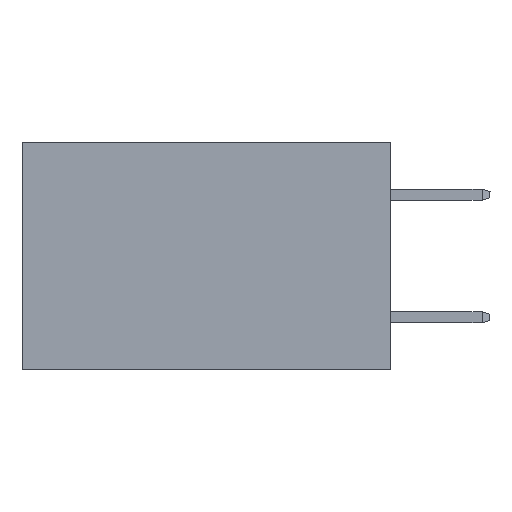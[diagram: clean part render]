
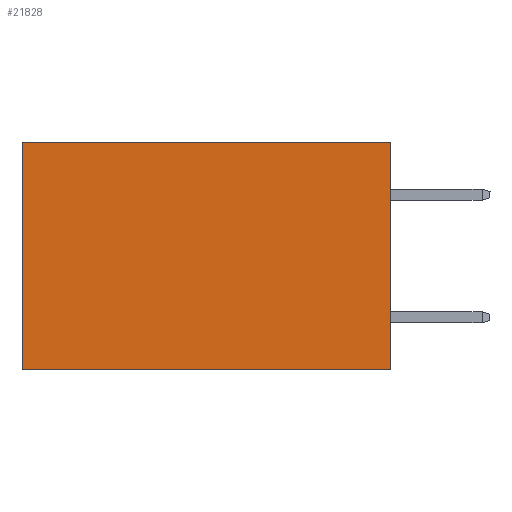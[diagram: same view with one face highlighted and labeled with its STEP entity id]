
A CAD part, left-side view. The second image highlights one B-rep face of the part: STEP entity #21828.
In plain terms, the highlighted planar face has unit normal (-1, 0, 0).
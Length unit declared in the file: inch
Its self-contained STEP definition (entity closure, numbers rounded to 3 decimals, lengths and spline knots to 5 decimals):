
#1459 = ORIENTED_EDGE ( 'NONE', *, *, #14825, .T. ) ;
#3562 = CARTESIAN_POINT ( 'NONE',  ( 0.2875, 0., 0. ) ) ;
#5300 = LINE ( 'NONE', #7454, #20309 ) ;
#5664 = DIRECTION ( 'NONE',  ( 0., 0., -1. ) ) ;
#5943 = ORIENTED_EDGE ( 'NONE', *, *, #11505, .F. ) ;
#6032 = CARTESIAN_POINT ( 'NONE',  ( 0.2875, 0.6, -0.37 ) ) ;
#6483 = LINE ( 'NONE', #3562, #21457 ) ;
#6856 = DIRECTION ( 'NONE',  ( 0., 1., 0. ) ) ;
#7454 = CARTESIAN_POINT ( 'NONE',  ( 0.2875, 0.6, 0. ) ) ;
#7782 = CARTESIAN_POINT ( 'NONE',  ( 0.2875, 0., 0. ) ) ;
#8153 = LINE ( 'NONE', #21104, #13631 ) ;
#8160 = PLANE ( 'NONE',  #14779 ) ;
#8751 = EDGE_LOOP ( 'NONE', ( #1459, #10236, #5943, #17348 ) ) ;
#9636 = DIRECTION ( 'NONE',  ( 0., 0., -1. ) ) ;
#9799 = FACE_OUTER_BOUND ( 'NONE', #8751, .T. ) ;
#10236 = ORIENTED_EDGE ( 'NONE', *, *, #22130, .F. ) ;
#10277 = CARTESIAN_POINT ( 'NONE',  ( 0.2875, 0., 0. ) ) ;
#11505 = EDGE_CURVE ( 'NONE', #23575, #16893, #24968, .T. ) ;
#12312 = DIRECTION ( 'NONE',  ( 1., 0., 0. ) ) ;
#13497 = EDGE_CURVE ( 'NONE', #23575, #19678, #6483, .T. ) ;
#13631 = VECTOR ( 'NONE', #6856, 39.37008 ) ;
#14385 = VECTOR ( 'NONE', #5664, 39.37008 ) ;
#14779 = AXIS2_PLACEMENT_3D ( 'NONE', #10277, #12312, #24291 ) ;
#14825 = EDGE_CURVE ( 'NONE', #19678, #26076, #5300, .T. ) ;
#16893 = VERTEX_POINT ( 'NONE', #25299 ) ;
#17348 = ORIENTED_EDGE ( 'NONE', *, *, #13497, .T. ) ;
#17731 = CARTESIAN_POINT ( 'NONE',  ( 0.2875, 0., 0. ) ) ;
#19678 = VERTEX_POINT ( 'NONE', #25683 ) ;
#19884 = DIRECTION ( 'NONE',  ( 0., 1., 0. ) ) ;
#20309 = VECTOR ( 'NONE', #9636, 39.37008 ) ;
#21104 = CARTESIAN_POINT ( 'NONE',  ( 0.2875, 0., -0.37 ) ) ;
#21457 = VECTOR ( 'NONE', #19884, 39.37008 ) ;
#21828 = ADVANCED_FACE ( 'NONE', ( #9799 ), #8160, .F. ) ;
#22130 = EDGE_CURVE ( 'NONE', #16893, #26076, #8153, .T. ) ;
#23575 = VERTEX_POINT ( 'NONE', #17731 ) ;
#24291 = DIRECTION ( 'NONE',  ( 0., 0., -1. ) ) ;
#24968 = LINE ( 'NONE', #7782, #14385 ) ;
#25299 = CARTESIAN_POINT ( 'NONE',  ( 0.2875, 0., -0.37 ) ) ;
#25683 = CARTESIAN_POINT ( 'NONE',  ( 0.2875, 0.6, 0. ) ) ;
#26076 = VERTEX_POINT ( 'NONE', #6032 ) ;
